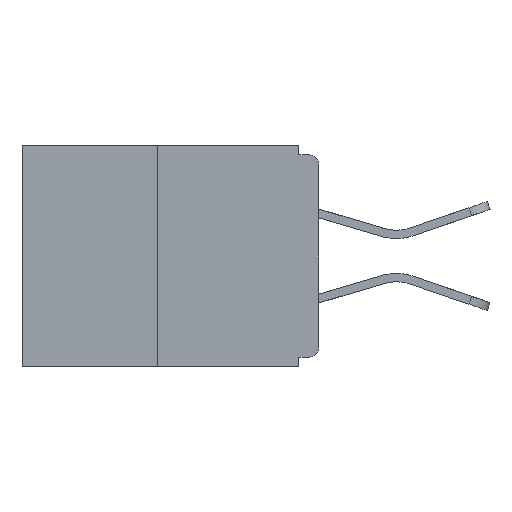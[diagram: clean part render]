
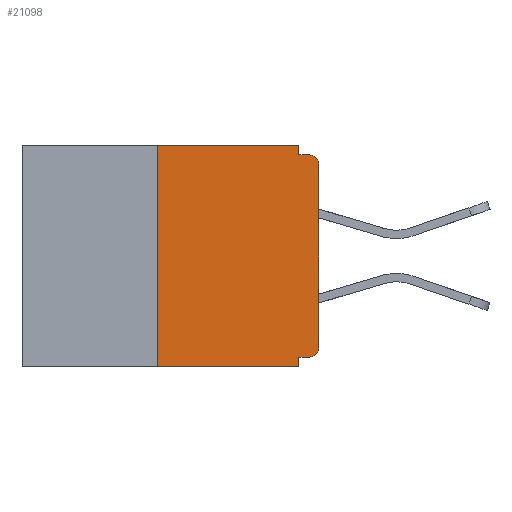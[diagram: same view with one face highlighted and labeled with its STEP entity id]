
A CAD part, left-side view. The second image highlights one B-rep face of the part: STEP entity #21098.
In plain terms, the highlighted planar face has unit normal (-1, 0, 0).
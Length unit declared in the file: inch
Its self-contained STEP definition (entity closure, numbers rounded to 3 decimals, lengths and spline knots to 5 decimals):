
#467 = VERTEX_POINT ( 'NONE', #5932 ) ;
#486 = ORIENTED_EDGE ( 'NONE', *, *, #22309, .F. ) ;
#588 = EDGE_CURVE ( 'NONE', #6334, #11463, #15449, .T. ) ;
#790 = EDGE_CURVE ( 'NONE', #3091, #12741, #10133, .T. ) ;
#1231 = DIRECTION ( 'NONE',  ( 1., 0., 0. ) ) ;
#1450 = VECTOR ( 'NONE', #12407, 39.37008 ) ;
#1989 = CARTESIAN_POINT ( 'NONE',  ( 0., 0.031, -0.343 ) ) ;
#2417 = ORIENTED_EDGE ( 'NONE', *, *, #23489, .F. ) ;
#2636 = LINE ( 'NONE', #17844, #3241 ) ;
#2646 = CARTESIAN_POINT ( 'NONE',  ( 0., 0.25, -0.343 ) ) ;
#2869 = CARTESIAN_POINT ( 'NONE',  ( 0., 0.031, -0.343 ) ) ;
#3091 = VERTEX_POINT ( 'NONE', #5362 ) ;
#3092 = EDGE_CURVE ( 'NONE', #12973, #14473, #20813, .T. ) ;
#3210 = DIRECTION ( 'NONE',  ( 0., 0., 1. ) ) ;
#3241 = VECTOR ( 'NONE', #15872, 39.37008 ) ;
#3359 = LINE ( 'NONE', #9028, #1450 ) ;
#3381 = CARTESIAN_POINT ( 'NONE',  ( 0., 0.25, 0. ) ) ;
#3747 = AXIS2_PLACEMENT_3D ( 'NONE', #16180, #12129, #21381 ) ;
#4068 = CARTESIAN_POINT ( 'NONE',  ( 0., 0.46, -0.343 ) ) ;
#4328 = VECTOR ( 'NONE', #19051, 39.37008 ) ;
#4833 = VERTEX_POINT ( 'NONE', #3381 ) ;
#5059 = LINE ( 'NONE', #22359, #7078 ) ;
#5173 = CARTESIAN_POINT ( 'NONE',  ( 0., 0.46, 0. ) ) ;
#5331 = EDGE_CURVE ( 'NONE', #8602, #11463, #17185, .T. ) ;
#5362 = CARTESIAN_POINT ( 'NONE',  ( 0., 0.031, 0. ) ) ;
#5548 = ORIENTED_EDGE ( 'NONE', *, *, #588, .T. ) ;
#5610 = EDGE_CURVE ( 'NONE', #467, #12973, #5059, .T. ) ;
#5932 = CARTESIAN_POINT ( 'NONE',  ( 0., 0., -0.313 ) ) ;
#6115 = AXIS2_PLACEMENT_3D ( 'NONE', #5173, #1231, #8751 ) ;
#6268 = VECTOR ( 'NONE', #6276, 39.37008 ) ;
#6276 = DIRECTION ( 'NONE',  ( 0., -1., 0. ) ) ;
#6334 = VERTEX_POINT ( 'NONE', #2646 ) ;
#7078 = VECTOR ( 'NONE', #3210, 39.37008 ) ;
#7165 = CARTESIAN_POINT ( 'NONE',  ( 0., 0.015, -0.015 ) ) ;
#7735 = EDGE_CURVE ( 'NONE', #14659, #8602, #2636, .T. ) ;
#7885 = EDGE_LOOP ( 'NONE', ( #21802, #486, #5548, #19486, #23114, #18939, #15337, #15280, #2417, #21153 ) ) ;
#8602 = VERTEX_POINT ( 'NONE', #9757 ) ;
#8751 = DIRECTION ( 'NONE',  ( 0., 0., -1. ) ) ;
#9028 = CARTESIAN_POINT ( 'NONE',  ( 0., 0.46, 0. ) ) ;
#9188 = CARTESIAN_POINT ( 'NONE',  ( 0., 0.015, -0.03 ) ) ;
#9757 = CARTESIAN_POINT ( 'NONE',  ( 0., 0.031, -0.328 ) ) ;
#10053 = CIRCLE ( 'NONE', #3747, 0.015 ) ;
#10133 = LINE ( 'NONE', #15817, #21839 ) ;
#11463 = VERTEX_POINT ( 'NONE', #2869 ) ;
#11923 = LINE ( 'NONE', #22767, #23474 ) ;
#12129 = DIRECTION ( 'NONE',  ( -1., 0., 0. ) ) ;
#12407 = DIRECTION ( 'NONE',  ( 0., -1., 0. ) ) ;
#12553 = AXIS2_PLACEMENT_3D ( 'NONE', #9188, #12559, #22295 ) ;
#12559 = DIRECTION ( 'NONE',  ( -1., 0., 0. ) ) ;
#12649 = EDGE_CURVE ( 'NONE', #14659, #467, #10053, .T. ) ;
#12741 = VERTEX_POINT ( 'NONE', #16060 ) ;
#12750 = FACE_OUTER_BOUND ( 'NONE', #7885, .T. ) ;
#12973 = VERTEX_POINT ( 'NONE', #21503 ) ;
#14473 = VERTEX_POINT ( 'NONE', #7165 ) ;
#14659 = VERTEX_POINT ( 'NONE', #19493 ) ;
#15268 = VECTOR ( 'NONE', #17661, 39.37008 ) ;
#15280 = ORIENTED_EDGE ( 'NONE', *, *, #3092, .T. ) ;
#15337 = ORIENTED_EDGE ( 'NONE', *, *, #5610, .T. ) ;
#15449 = LINE ( 'NONE', #4068, #6268 ) ;
#15817 = CARTESIAN_POINT ( 'NONE',  ( 0., 0.031, 0. ) ) ;
#15872 = DIRECTION ( 'NONE',  ( 0., 1., 0. ) ) ;
#16060 = CARTESIAN_POINT ( 'NONE',  ( 0., 0.031, -0.015 ) ) ;
#16180 = CARTESIAN_POINT ( 'NONE',  ( 0., 0.015, -0.313 ) ) ;
#17185 = LINE ( 'NONE', #1989, #4328 ) ;
#17297 = CARTESIAN_POINT ( 'NONE',  ( 0., 0.25, 0. ) ) ;
#17542 = LINE ( 'NONE', #17297, #15268 ) ;
#17661 = DIRECTION ( 'NONE',  ( 0., 0., 1. ) ) ;
#17844 = CARTESIAN_POINT ( 'NONE',  ( 0., 0., -0.328 ) ) ;
#18939 = ORIENTED_EDGE ( 'NONE', *, *, #12649, .T. ) ;
#19051 = DIRECTION ( 'NONE',  ( 0., 0., -1. ) ) ;
#19486 = ORIENTED_EDGE ( 'NONE', *, *, #5331, .F. ) ;
#19493 = CARTESIAN_POINT ( 'NONE',  ( 0., 0.015, -0.328 ) ) ;
#20813 = CIRCLE ( 'NONE', #12553, 0.015 ) ;
#21098 = ADVANCED_FACE ( 'NONE', ( #12750 ), #22113, .F. ) ;
#21153 = ORIENTED_EDGE ( 'NONE', *, *, #790, .F. ) ;
#21381 = DIRECTION ( 'NONE',  ( 0., 0., -1. ) ) ;
#21503 = CARTESIAN_POINT ( 'NONE',  ( 0., 0., -0.03 ) ) ;
#21802 = ORIENTED_EDGE ( 'NONE', *, *, #22029, .F. ) ;
#21839 = VECTOR ( 'NONE', #23345, 39.37008 ) ;
#22029 = EDGE_CURVE ( 'NONE', #4833, #3091, #3359, .T. ) ;
#22113 = PLANE ( 'NONE',  #6115 ) ;
#22295 = DIRECTION ( 'NONE',  ( 0., 0., -1. ) ) ;
#22309 = EDGE_CURVE ( 'NONE', #6334, #4833, #17542, .T. ) ;
#22359 = CARTESIAN_POINT ( 'NONE',  ( 0., 0., 0. ) ) ;
#22655 = DIRECTION ( 'NONE',  ( 0., -1., 0. ) ) ;
#22767 = CARTESIAN_POINT ( 'NONE',  ( 0., 0., -0.015 ) ) ;
#23114 = ORIENTED_EDGE ( 'NONE', *, *, #7735, .F. ) ;
#23345 = DIRECTION ( 'NONE',  ( 0., 0., -1. ) ) ;
#23474 = VECTOR ( 'NONE', #22655, 39.37008 ) ;
#23489 = EDGE_CURVE ( 'NONE', #12741, #14473, #11923, .T. ) ;
